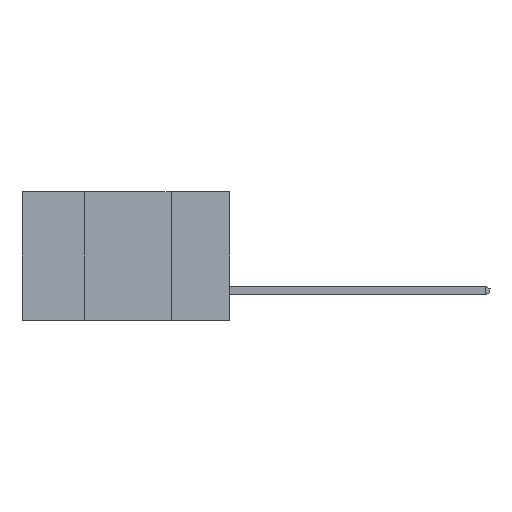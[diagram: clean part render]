
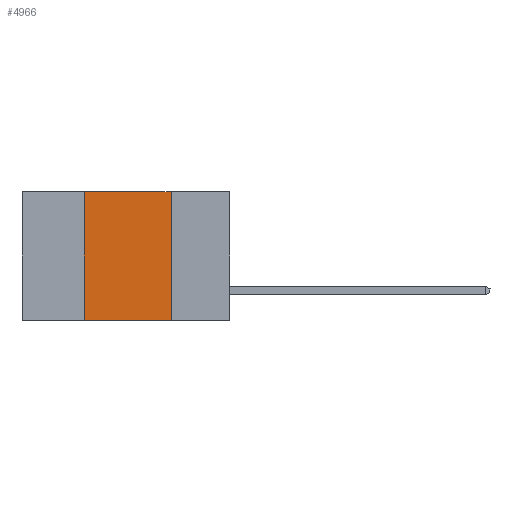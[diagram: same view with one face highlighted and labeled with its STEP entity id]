
A CAD part, left-side view. The second image highlights one B-rep face of the part: STEP entity #4966.
In plain terms, the highlighted planar face has unit normal (-1, 0, 0).
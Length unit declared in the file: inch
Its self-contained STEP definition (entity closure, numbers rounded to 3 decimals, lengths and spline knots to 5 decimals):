
#193 = CARTESIAN_POINT ( 'NONE',  ( 0., 0.6, 0. ) ) ;
#438 = ORIENTED_EDGE ( 'NONE', *, *, #1888, .F. ) ;
#587 = CARTESIAN_POINT ( 'NONE',  ( 0., 0.42, -0.37 ) ) ;
#674 = ORIENTED_EDGE ( 'NONE', *, *, #9325, .F. ) ;
#732 = EDGE_CURVE ( 'NONE', #3543, #4485, #9171, .T. ) ;
#1169 = DIRECTION ( 'NONE',  ( 0., 0., -1. ) ) ;
#1276 = AXIS2_PLACEMENT_3D ( 'NONE', #6824, #5268, #1169 ) ;
#1315 = ORIENTED_EDGE ( 'NONE', *, *, #732, .F. ) ;
#1656 = EDGE_LOOP ( 'NONE', ( #674, #1315, #438, #5803 ) ) ;
#1737 = DIRECTION ( 'NONE',  ( 0., -1., 0. ) ) ;
#1888 = EDGE_CURVE ( 'NONE', #4891, #3543, #7254, .T. ) ;
#1982 = PLANE ( 'NONE',  #1276 ) ;
#2126 = LINE ( 'NONE', #5414, #7189 ) ;
#2795 = FACE_OUTER_BOUND ( 'NONE', #1656, .T. ) ;
#3537 = CARTESIAN_POINT ( 'NONE',  ( 0., 0.17, -0.37 ) ) ;
#3543 = VERTEX_POINT ( 'NONE', #8124 ) ;
#4370 = CARTESIAN_POINT ( 'NONE',  ( 0., 0.17, 0. ) ) ;
#4409 = CARTESIAN_POINT ( 'NONE',  ( 0., 0.42, -0.37 ) ) ;
#4485 = VERTEX_POINT ( 'NONE', #4370 ) ;
#4730 = CARTESIAN_POINT ( 'NONE',  ( 0., 0.17, -0.37 ) ) ;
#4891 = VERTEX_POINT ( 'NONE', #4409 ) ;
#4966 = ADVANCED_FACE ( 'NONE', ( #2795 ), #1982, .F. ) ;
#5229 = DIRECTION ( 'NONE',  ( 0., 0., -1. ) ) ;
#5268 = DIRECTION ( 'NONE',  ( 1., 0., 0. ) ) ;
#5414 = CARTESIAN_POINT ( 'NONE',  ( 0., 0.6, -0.37 ) ) ;
#5585 = LINE ( 'NONE', #4730, #9299 ) ;
#5803 = ORIENTED_EDGE ( 'NONE', *, *, #7344, .T. ) ;
#6824 = CARTESIAN_POINT ( 'NONE',  ( 0., 0.6, 0. ) ) ;
#6855 = VECTOR ( 'NONE', #8018, 39.37008 ) ;
#7189 = VECTOR ( 'NONE', #7878, 39.37008 ) ;
#7254 = LINE ( 'NONE', #587, #6855 ) ;
#7344 = EDGE_CURVE ( 'NONE', #4891, #8425, #2126, .T. ) ;
#7878 = DIRECTION ( 'NONE',  ( 0., -1., 0. ) ) ;
#8018 = DIRECTION ( 'NONE',  ( 0., 0., 1. ) ) ;
#8124 = CARTESIAN_POINT ( 'NONE',  ( 0., 0.42, 0. ) ) ;
#8425 = VERTEX_POINT ( 'NONE', #3537 ) ;
#8780 = VECTOR ( 'NONE', #1737, 39.37008 ) ;
#9171 = LINE ( 'NONE', #193, #8780 ) ;
#9299 = VECTOR ( 'NONE', #5229, 39.37008 ) ;
#9325 = EDGE_CURVE ( 'NONE', #4485, #8425, #5585, .T. ) ;
